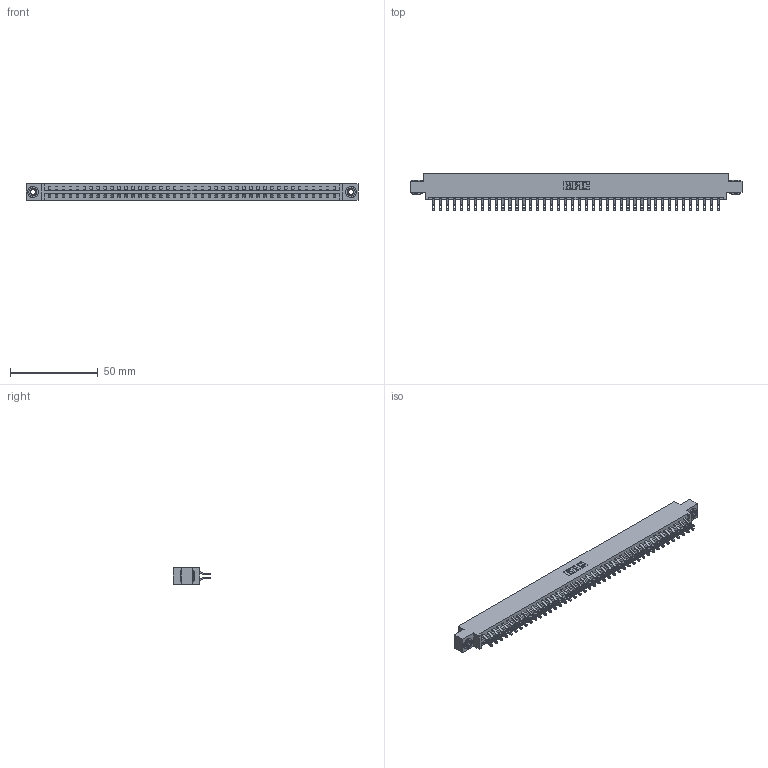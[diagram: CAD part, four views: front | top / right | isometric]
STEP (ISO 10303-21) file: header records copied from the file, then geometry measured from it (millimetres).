
FILE_DESCRIPTION (( 'STEP AP203' ), '1' );
FILE_NAME ('337-084-555-803.STEP', '2019-10-15T18:15:55', ( '' ), ( '' ), 'SwSTEP 2.0', 'SolidWorks 2016', '' );
FILE_SCHEMA (( 'CONFIG_CONTROL_DESIGN' ));
Length unit declared in the file: inch
Products named in the file (4): 345-250-002_345-250-002-102; 345-292-001_555 Tail; 337 Part_0.170 Offset - 0.156 Dia-TH; 337-084-555-803
Assembly tree (87 placements, depth 2):
  337-084-555-803
    337 Part_0.170 Offset - 0.156 Dia-TH
    345-292-001_555 Tail  x84
    345-250-002_345-250-002-102  x2
Bounding box: 189.43 x 21.47 x 9.4 mm (x, y, z)
Volume: 20109.5 mm3; surface area: 23984.3 mm2
Topology: 87 solids, 87 shells, 5196 faces, 16275 edges, 10846 vertices
Faces by surface type: plane 3108, cylinder 2080, cone 8
Entity records: 33672 total; most frequent: CARTESIAN_POINT 5683, ORIENTED_EDGE 5582, DIRECTION 4837, EDGE_CURVE 2791, VECTOR 2619, LINE 2619, VERTEX_POINT 1858, AXIS2_PLACEMENT_3D 1109
